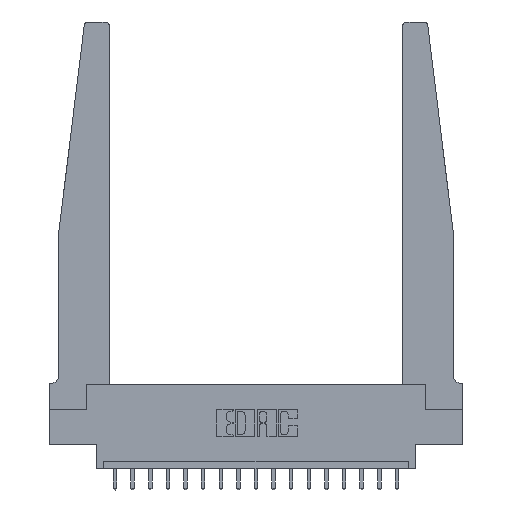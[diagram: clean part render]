
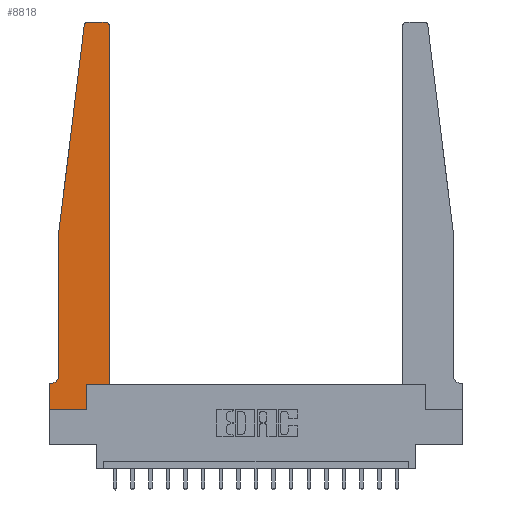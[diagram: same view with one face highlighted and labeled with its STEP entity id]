
A CAD part, top view. The second image highlights one B-rep face of the part: STEP entity #8818.
In plain terms, the highlighted planar face has unit normal (0, 0, 1).
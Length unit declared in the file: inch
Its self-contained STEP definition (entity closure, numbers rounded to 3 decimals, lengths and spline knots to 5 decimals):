
#153 = PLANE ( 'NONE',  #8485 ) ;
#424 = ORIENTED_EDGE ( 'NONE', *, *, #626, .T. ) ;
#436 = DIRECTION ( 'NONE',  ( 1., 0., 0. ) ) ;
#514 = CARTESIAN_POINT ( 'NONE',  ( 0., 0., 0.37 ) ) ;
#578 = LINE ( 'NONE', #11432, #15624 ) ;
#626 = EDGE_CURVE ( 'NONE', #9671, #6825, #1804, .T. ) ;
#879 = ORIENTED_EDGE ( 'NONE', *, *, #8838, .T. ) ;
#1378 = ORIENTED_EDGE ( 'NONE', *, *, #10819, .T. ) ;
#1436 = CIRCLE ( 'NONE', #17871, 0.05 ) ;
#1523 = DIRECTION ( 'NONE',  ( 0., -1., 0. ) ) ;
#1573 = EDGE_CURVE ( 'NONE', #14662, #9229, #4649, .T. ) ;
#1804 = CIRCLE ( 'NONE', #18048, 0.03 ) ;
#2074 = DIRECTION ( 'NONE',  ( -1., 0., 0. ) ) ;
#2081 = CARTESIAN_POINT ( 'NONE',  ( 0.425, 0.18, 0.37 ) ) ;
#2812 = ORIENTED_EDGE ( 'NONE', *, *, #10326, .T. ) ;
#2836 = VERTEX_POINT ( 'NONE', #18751 ) ;
#3040 = FACE_OUTER_BOUND ( 'NONE', #14065, .T. ) ;
#3066 = DIRECTION ( 'NONE',  ( 1., 0., 0. ) ) ;
#3539 = CARTESIAN_POINT ( 'NONE',  ( 0.395, 2.72, 0.37 ) ) ;
#3956 = EDGE_CURVE ( 'NONE', #8723, #14662, #7492, .T. ) ;
#4001 = CARTESIAN_POINT ( 'NONE',  ( 0.24675, 2.72367, 0.37 ) ) ;
#4359 = CARTESIAN_POINT ( 'NONE',  ( 0.395, 2.75, 0.37 ) ) ;
#4557 = CARTESIAN_POINT ( 'NONE',  ( 0.25, 2.75, 0.37 ) ) ;
#4643 = CARTESIAN_POINT ( 'NONE',  ( 0., 0., 0.37 ) ) ;
#4649 = LINE ( 'NONE', #4643, #16705 ) ;
#4740 = VERTEX_POINT ( 'NONE', #5435 ) ;
#5060 = VECTOR ( 'NONE', #7724, 39.37008 ) ;
#5297 = DIRECTION ( 'NONE',  ( 1., 0., 0. ) ) ;
#5435 = CARTESIAN_POINT ( 'NONE',  ( 0.27653, 2.75, 0.37 ) ) ;
#5827 = ORIENTED_EDGE ( 'NONE', *, *, #3956, .T. ) ;
#6070 = DIRECTION ( 'NONE',  ( -1., 0., 0. ) ) ;
#6553 = EDGE_CURVE ( 'NONE', #15638, #2836, #13588, .T. ) ;
#6618 = ORIENTED_EDGE ( 'NONE', *, *, #8758, .T. ) ;
#6624 = VECTOR ( 'NONE', #17074, 39.37008 ) ;
#6697 = LINE ( 'NONE', #4557, #13526 ) ;
#6825 = VERTEX_POINT ( 'NONE', #4359 ) ;
#7264 = LINE ( 'NONE', #16647, #17900 ) ;
#7492 = LINE ( 'NONE', #514, #15273 ) ;
#7630 = DIRECTION ( 'NONE',  ( -1., 0., 0. ) ) ;
#7724 = DIRECTION ( 'NONE',  ( -0.122, -0.992, 0. ) ) ;
#7863 = CARTESIAN_POINT ( 'NONE',  ( 0.065, 0.1875, 0.37 ) ) ;
#7865 = DIRECTION ( 'NONE',  ( 0., 1., 0. ) ) ;
#8185 = EDGE_CURVE ( 'NONE', #4740, #16740, #9184, .T. ) ;
#8429 = EDGE_CURVE ( 'NONE', #11458, #8723, #15369, .T. ) ;
#8485 = AXIS2_PLACEMENT_3D ( 'NONE', #13076, #10315, #3066 ) ;
#8510 = VECTOR ( 'NONE', #2074, 39.37008 ) ;
#8518 = ORIENTED_EDGE ( 'NONE', *, *, #14592, .T. ) ;
#8723 = VERTEX_POINT ( 'NONE', #17433 ) ;
#8758 = EDGE_CURVE ( 'NONE', #2836, #11458, #1436, .T. ) ;
#8761 = CARTESIAN_POINT ( 'NONE',  ( 0.065, 1.25, 0.37 ) ) ;
#8778 = CARTESIAN_POINT ( 'NONE',  ( 0.015, 0.2375, 0.37 ) ) ;
#8818 = ADVANCED_FACE ( 'NONE', ( #3040 ), #153, .T. ) ;
#8838 = EDGE_CURVE ( 'NONE', #6825, #4740, #6697, .T. ) ;
#9184 = CIRCLE ( 'NONE', #15830, 0.03 ) ;
#9229 = VERTEX_POINT ( 'NONE', #16978 ) ;
#9580 = CARTESIAN_POINT ( 'NONE',  ( 0.065, 1.25, 0.37 ) ) ;
#9671 = VERTEX_POINT ( 'NONE', #13685 ) ;
#10315 = DIRECTION ( 'NONE',  ( 0., 0., 1. ) ) ;
#10326 = EDGE_CURVE ( 'NONE', #16740, #15638, #18234, .T. ) ;
#10416 = DIRECTION ( 'NONE',  ( 0., 0., 1. ) ) ;
#10435 = DIRECTION ( 'NONE',  ( 0., -1., 0. ) ) ;
#10551 = DIRECTION ( 'NONE',  ( 1., 0., 0. ) ) ;
#10819 = EDGE_CURVE ( 'NONE', #11590, #14162, #16635, .T. ) ;
#10982 = ORIENTED_EDGE ( 'NONE', *, *, #8185, .T. ) ;
#11213 = DIRECTION ( 'NONE',  ( 0., 0., 1. ) ) ;
#11432 = CARTESIAN_POINT ( 'NONE',  ( 0.425, 0.18, 0.37 ) ) ;
#11458 = VERTEX_POINT ( 'NONE', #16426 ) ;
#11590 = VERTEX_POINT ( 'NONE', #12561 ) ;
#11755 = ORIENTED_EDGE ( 'NONE', *, *, #6553, .T. ) ;
#11853 = ORIENTED_EDGE ( 'NONE', *, *, #1573, .T. ) ;
#12561 = CARTESIAN_POINT ( 'NONE',  ( 0.2605, 0.18, 0.37 ) ) ;
#12657 = ORIENTED_EDGE ( 'NONE', *, *, #15225, .T. ) ;
#13076 = CARTESIAN_POINT ( 'NONE',  ( 0., 0.1875, 0.37 ) ) ;
#13363 = CARTESIAN_POINT ( 'NONE',  ( 0., 0., 0.37 ) ) ;
#13526 = VECTOR ( 'NONE', #7630, 39.37008 ) ;
#13588 = LINE ( 'NONE', #8761, #18132 ) ;
#13685 = CARTESIAN_POINT ( 'NONE',  ( 0.425, 2.72, 0.37 ) ) ;
#14065 = EDGE_LOOP ( 'NONE', ( #879, #10982, #2812, #11755, #6618, #14951, #5827, #11853, #12657, #1378, #8518, #424 ) ) ;
#14162 = VERTEX_POINT ( 'NONE', #2081 ) ;
#14592 = EDGE_CURVE ( 'NONE', #14162, #9671, #578, .T. ) ;
#14662 = VERTEX_POINT ( 'NONE', #13363 ) ;
#14951 = ORIENTED_EDGE ( 'NONE', *, *, #8429, .T. ) ;
#15225 = EDGE_CURVE ( 'NONE', #9229, #11590, #7264, .T. ) ;
#15256 = CARTESIAN_POINT ( 'NONE',  ( 0.065, 1.25, 0.37 ) ) ;
#15273 = VECTOR ( 'NONE', #10435, 39.37008 ) ;
#15346 = DIRECTION ( 'NONE',  ( 0., 1., 0. ) ) ;
#15369 = LINE ( 'NONE', #7863, #8510 ) ;
#15587 = CARTESIAN_POINT ( 'NONE',  ( 0.425, 0.18, 0.37 ) ) ;
#15624 = VECTOR ( 'NONE', #15346, 39.37008 ) ;
#15638 = VERTEX_POINT ( 'NONE', #9580 ) ;
#15830 = AXIS2_PLACEMENT_3D ( 'NONE', #16456, #10416, #436 ) ;
#16426 = CARTESIAN_POINT ( 'NONE',  ( 0.015, 0.1875, 0.37 ) ) ;
#16456 = CARTESIAN_POINT ( 'NONE',  ( 0.27653, 2.72, 0.37 ) ) ;
#16635 = LINE ( 'NONE', #15587, #6624 ) ;
#16647 = CARTESIAN_POINT ( 'NONE',  ( 0.2605, 0.18, 0.37 ) ) ;
#16705 = VECTOR ( 'NONE', #10551, 39.37008 ) ;
#16740 = VERTEX_POINT ( 'NONE', #4001 ) ;
#16978 = CARTESIAN_POINT ( 'NONE',  ( 0.2605, 0., 0.37 ) ) ;
#17074 = DIRECTION ( 'NONE',  ( 1., 0., 0. ) ) ;
#17433 = CARTESIAN_POINT ( 'NONE',  ( 0., 0.1875, 0.37 ) ) ;
#17497 = DIRECTION ( 'NONE',  ( 0., 0., -1. ) ) ;
#17871 = AXIS2_PLACEMENT_3D ( 'NONE', #8778, #17497, #6070 ) ;
#17900 = VECTOR ( 'NONE', #7865, 39.37008 ) ;
#18048 = AXIS2_PLACEMENT_3D ( 'NONE', #3539, #11213, #5297 ) ;
#18132 = VECTOR ( 'NONE', #1523, 39.37008 ) ;
#18234 = LINE ( 'NONE', #15256, #5060 ) ;
#18751 = CARTESIAN_POINT ( 'NONE',  ( 0.065, 0.2375, 0.37 ) ) ;
